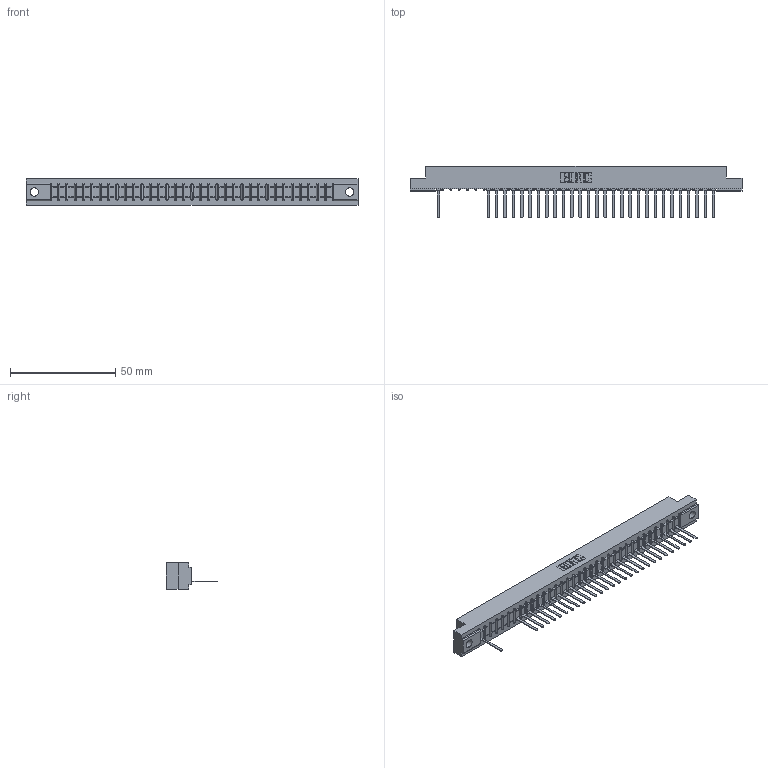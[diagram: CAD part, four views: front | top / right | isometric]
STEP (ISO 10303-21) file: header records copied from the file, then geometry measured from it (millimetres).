
FILE_DESCRIPTION (( 'STEP AP203' ), '1' );
FILE_NAME ('357-034-541-104.STEP', '2018-08-10T02:35:50', ( '' ), ( '' ), 'SwSTEP 2.0', 'SolidWorks 2016', '' );
FILE_SCHEMA (( 'CONFIG_CONTROL_DESIGN' ));
Length unit declared in the file: inch
Products named in the file (3): 307 Part_.156 Dia Mounting Holes; 307-290-002_541; 357-034-541-104
Assembly tree (30 placements, depth 2):
  357-034-541-104
    307 Part_.156 Dia Mounting Holes
    307-290-002_541  x29
Bounding box: 157.73 x 24.59 x 12.7 mm (x, y, z)
Volume: 16651.1 mm3; surface area: 20197 mm2
Topology: 30 solids, 30 shells, 2413 faces, 7407 edges, 4842 vertices
Faces by surface type: plane 1449, cylinder 894, sphere 70
Entity records: 31110 total; most frequent: CARTESIAN_POINT 5273, ORIENTED_EDGE 5266, DIRECTION 5113, EDGE_CURVE 2633, VECTOR 2021, LINE 2021, VERTEX_POINT 1706, AXIS2_PLACEMENT_3D 1546
